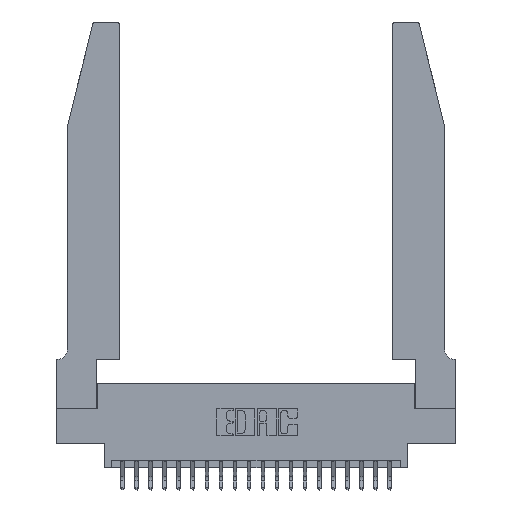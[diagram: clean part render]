
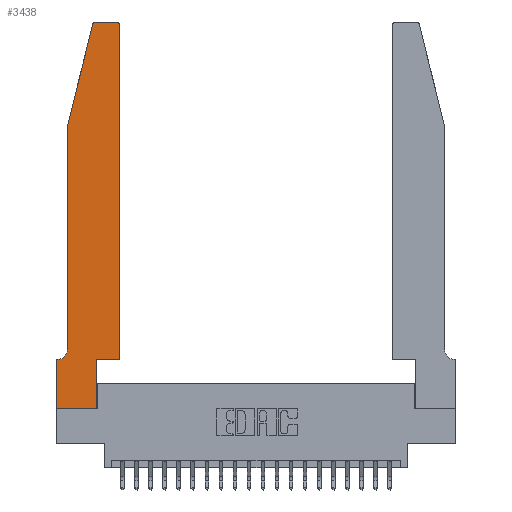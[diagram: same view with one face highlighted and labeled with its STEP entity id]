
A CAD part, top view. The second image highlights one B-rep face of the part: STEP entity #3438.
In plain terms, the highlighted planar face has unit normal (0, 0, 1).
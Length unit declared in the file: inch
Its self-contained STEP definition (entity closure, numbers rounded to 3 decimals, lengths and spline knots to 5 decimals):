
#76 = CARTESIAN_POINT ( 'NONE',  ( 0.4505, 0.35, 0.37 ) ) ;
#204 = VERTEX_POINT ( 'NONE', #16984 ) ;
#635 = DIRECTION ( 'NONE',  ( -1., 0., 0. ) ) ;
#815 = DIRECTION ( 'NONE',  ( -1., 0., 0. ) ) ;
#825 = LINE ( 'NONE', #2510, #5740 ) ;
#894 = CARTESIAN_POINT ( 'NONE',  ( 0.0055, 0.42, 0.37 ) ) ;
#1231 = ORIENTED_EDGE ( 'NONE', *, *, #15978, .T. ) ;
#1407 = CARTESIAN_POINT ( 'NONE',  ( 0.2865, 0., 0.37 ) ) ;
#1690 = VECTOR ( 'NONE', #20099, 39.37008 ) ;
#2225 = CIRCLE ( 'NONE', #9771, 0.07 ) ;
#2248 = EDGE_CURVE ( 'NONE', #21944, #8605, #4915, .T. ) ;
#2510 = CARTESIAN_POINT ( 'NONE',  ( 0.2605, 2.75, 0.37 ) ) ;
#2631 = DIRECTION ( 'NONE',  ( 0., 0., 1. ) ) ;
#3132 = DIRECTION ( 'NONE',  ( 0., 1., 0. ) ) ;
#3410 = DIRECTION ( 'NONE',  ( 1., 0., 0. ) ) ;
#3438 = ADVANCED_FACE ( 'NONE', ( #22930 ), #22619, .T. ) ;
#4161 = ORIENTED_EDGE ( 'NONE', *, *, #10732, .T. ) ;
#4163 = DIRECTION ( 'NONE',  ( 1., 0., 0. ) ) ;
#4230 = CARTESIAN_POINT ( 'NONE',  ( 0.4205, 2.75, 0.37 ) ) ;
#4251 = EDGE_CURVE ( 'NONE', #4368, #13360, #17736, .T. ) ;
#4290 = LINE ( 'NONE', #10950, #10295 ) ;
#4349 = AXIS2_PLACEMENT_3D ( 'NONE', #11924, #20841, #15629 ) ;
#4368 = VERTEX_POINT ( 'NONE', #9368 ) ;
#4915 = CIRCLE ( 'NONE', #7275, 0.03 ) ;
#5300 = CARTESIAN_POINT ( 'NONE',  ( 0.0755, 2., 0.37 ) ) ;
#5304 = ORIENTED_EDGE ( 'NONE', *, *, #15067, .T. ) ;
#5740 = VECTOR ( 'NONE', #635, 39.37008 ) ;
#5893 = EDGE_CURVE ( 'NONE', #13360, #204, #8743, .T. ) ;
#5967 = CARTESIAN_POINT ( 'NONE',  ( 0.0755, 2., 0.37 ) ) ;
#6440 = LINE ( 'NONE', #8878, #15296 ) ;
#7160 = ORIENTED_EDGE ( 'NONE', *, *, #2248, .T. ) ;
#7275 = AXIS2_PLACEMENT_3D ( 'NONE', #20147, #21940, #18456 ) ;
#7676 = EDGE_CURVE ( 'NONE', #19844, #11515, #10143, .T. ) ;
#8248 = CARTESIAN_POINT ( 'NONE',  ( 0.0755, 0.42, 0.37 ) ) ;
#8526 = VECTOR ( 'NONE', #3410, 39.37008 ) ;
#8605 = VERTEX_POINT ( 'NONE', #4230 ) ;
#8743 = LINE ( 'NONE', #23372, #10480 ) ;
#8878 = CARTESIAN_POINT ( 'NONE',  ( 0.4505, 0.35, 0.37 ) ) ;
#9121 = AXIS2_PLACEMENT_3D ( 'NONE', #9923, #2631, #4163 ) ;
#9171 = DIRECTION ( 'NONE',  ( 0., -1., 0. ) ) ;
#9368 = CARTESIAN_POINT ( 'NONE',  ( 0., 0., 0.37 ) ) ;
#9771 = AXIS2_PLACEMENT_3D ( 'NONE', #894, #11793, #815 ) ;
#9777 = VERTEX_POINT ( 'NONE', #19770 ) ;
#9923 = CARTESIAN_POINT ( 'NONE',  ( 0., 0.35, 0.37 ) ) ;
#10143 = LINE ( 'NONE', #13933, #21049 ) ;
#10162 = ORIENTED_EDGE ( 'NONE', *, *, #5893, .T. ) ;
#10295 = VECTOR ( 'NONE', #9171, 39.37008 ) ;
#10480 = VECTOR ( 'NONE', #15738, 39.37008 ) ;
#10662 = DIRECTION ( 'NONE',  ( -1., 0., 0. ) ) ;
#10732 = EDGE_CURVE ( 'NONE', #11515, #4368, #4290, .T. ) ;
#10950 = CARTESIAN_POINT ( 'NONE',  ( 0., 0., 0.37 ) ) ;
#11112 = ORIENTED_EDGE ( 'NONE', *, *, #18409, .T. ) ;
#11264 = VECTOR ( 'NONE', #20447, 39.37008 ) ;
#11515 = VERTEX_POINT ( 'NONE', #22221 ) ;
#11555 = ORIENTED_EDGE ( 'NONE', *, *, #22989, .T. ) ;
#11578 = ORIENTED_EDGE ( 'NONE', *, *, #19239, .T. ) ;
#11793 = DIRECTION ( 'NONE',  ( 0., 0., -1. ) ) ;
#11924 = CARTESIAN_POINT ( 'NONE',  ( 0.284, 2.72, 0.37 ) ) ;
#12043 = LINE ( 'NONE', #5300, #1690 ) ;
#13360 = VERTEX_POINT ( 'NONE', #1407 ) ;
#13467 = VERTEX_POINT ( 'NONE', #19425 ) ;
#13689 = CARTESIAN_POINT ( 'NONE',  ( 0.0055, 0.35, 0.37 ) ) ;
#13807 = ORIENTED_EDGE ( 'NONE', *, *, #19707, .T. ) ;
#13925 = VERTEX_POINT ( 'NONE', #8248 ) ;
#13933 = CARTESIAN_POINT ( 'NONE',  ( 0.0755, 0.35, 0.37 ) ) ;
#14589 = DIRECTION ( 'NONE',  ( 1., 0., 0. ) ) ;
#15067 = EDGE_CURVE ( 'NONE', #13467, #17241, #17295, .T. ) ;
#15296 = VECTOR ( 'NONE', #3132, 39.37008 ) ;
#15629 = DIRECTION ( 'NONE',  ( 1., 0., 0. ) ) ;
#15651 = CARTESIAN_POINT ( 'NONE',  ( 0.0755, 2., 0.37 ) ) ;
#15738 = DIRECTION ( 'NONE',  ( 0., 1., 0. ) ) ;
#15867 = ORIENTED_EDGE ( 'NONE', *, *, #20384, .T. ) ;
#15978 = EDGE_CURVE ( 'NONE', #9777, #13467, #17227, .T. ) ;
#16222 = CARTESIAN_POINT ( 'NONE',  ( 0.4505, 0.35, 0.37 ) ) ;
#16507 = ORIENTED_EDGE ( 'NONE', *, *, #4251, .T. ) ;
#16984 = CARTESIAN_POINT ( 'NONE',  ( 0.2865, 0.35, 0.37 ) ) ;
#17227 = CIRCLE ( 'NONE', #4349, 0.03 ) ;
#17241 = VERTEX_POINT ( 'NONE', #15651 ) ;
#17295 = LINE ( 'NONE', #5967, #11264 ) ;
#17523 = CARTESIAN_POINT ( 'NONE',  ( 0.4505, 2.72, 0.37 ) ) ;
#17736 = LINE ( 'NONE', #20056, #18867 ) ;
#18254 = EDGE_LOOP ( 'NONE', ( #13807, #1231, #5304, #11578, #15867, #20020, #4161, #16507, #10162, #11112, #11555, #7160 ) ) ;
#18409 = EDGE_CURVE ( 'NONE', #204, #23779, #19982, .T. ) ;
#18456 = DIRECTION ( 'NONE',  ( 1., 0., 0. ) ) ;
#18867 = VECTOR ( 'NONE', #14589, 39.37008 ) ;
#19239 = EDGE_CURVE ( 'NONE', #17241, #13925, #12043, .T. ) ;
#19425 = CARTESIAN_POINT ( 'NONE',  ( 0.25487, 2.72718, 0.37 ) ) ;
#19707 = EDGE_CURVE ( 'NONE', #8605, #9777, #825, .T. ) ;
#19770 = CARTESIAN_POINT ( 'NONE',  ( 0.284, 2.75, 0.37 ) ) ;
#19844 = VERTEX_POINT ( 'NONE', #13689 ) ;
#19982 = LINE ( 'NONE', #16222, #8526 ) ;
#20020 = ORIENTED_EDGE ( 'NONE', *, *, #7676, .T. ) ;
#20056 = CARTESIAN_POINT ( 'NONE',  ( 0., 0., 0.37 ) ) ;
#20099 = DIRECTION ( 'NONE',  ( 0., -1., 0. ) ) ;
#20147 = CARTESIAN_POINT ( 'NONE',  ( 0.4205, 2.72, 0.37 ) ) ;
#20384 = EDGE_CURVE ( 'NONE', #13925, #19844, #2225, .T. ) ;
#20447 = DIRECTION ( 'NONE',  ( -0.239, -0.971, 0. ) ) ;
#20841 = DIRECTION ( 'NONE',  ( 0., 0., 1. ) ) ;
#21049 = VECTOR ( 'NONE', #10662, 39.37008 ) ;
#21940 = DIRECTION ( 'NONE',  ( 0., 0., 1. ) ) ;
#21944 = VERTEX_POINT ( 'NONE', #17523 ) ;
#22221 = CARTESIAN_POINT ( 'NONE',  ( 0., 0.35, 0.37 ) ) ;
#22619 = PLANE ( 'NONE',  #9121 ) ;
#22930 = FACE_OUTER_BOUND ( 'NONE', #18254, .T. ) ;
#22989 = EDGE_CURVE ( 'NONE', #23779, #21944, #6440, .T. ) ;
#23372 = CARTESIAN_POINT ( 'NONE',  ( 0.2865, 0.35, 0.37 ) ) ;
#23779 = VERTEX_POINT ( 'NONE', #76 ) ;
